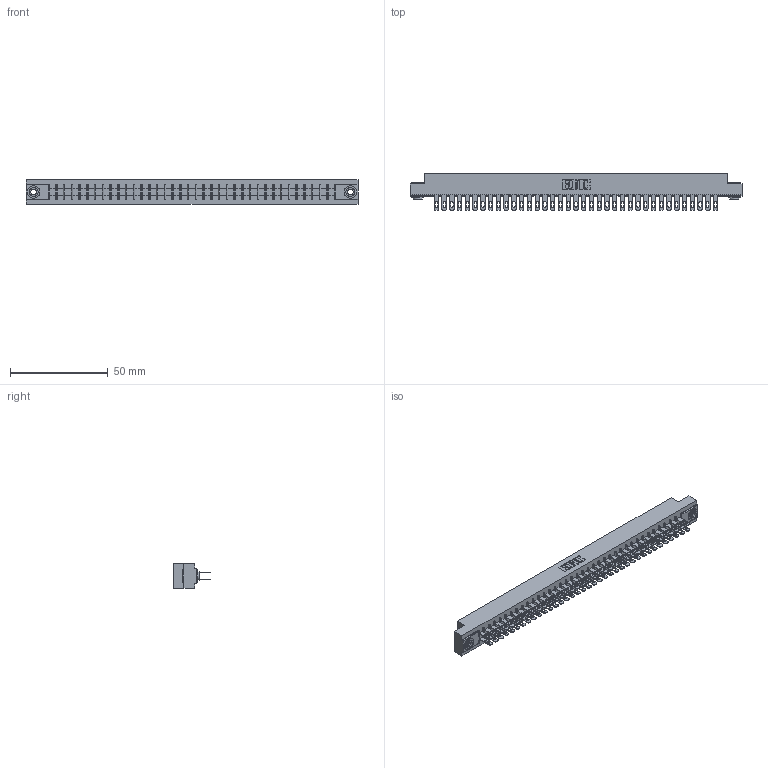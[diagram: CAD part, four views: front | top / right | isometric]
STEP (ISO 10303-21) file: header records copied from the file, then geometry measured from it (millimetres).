
FILE_DESCRIPTION (( 'STEP AP203' ), '1' );
FILE_NAME ('315-074-500-203.STEP', '2019-09-10T21:59:41', ( '' ), ( '' ), 'SwSTEP 2.0', 'SolidWorks 2016', '' );
FILE_SCHEMA (( 'CONFIG_CONTROL_DESIGN' ));
Length unit declared in the file: inch
Products named in the file (4): 305 Part_.156 Dia; 345-250-002_345-250-002-102; 305-290-001_500; 315-074-500-203
Assembly tree (77 placements, depth 2):
  315-074-500-203
    305 Part_.156 Dia
    305-290-001_500  x74
    345-250-002_345-250-002-102  x2
Bounding box: 169.62 x 18.85 x 12.7 mm (x, y, z)
Volume: 17897.6 mm3; surface area: 24349.3 mm2
Topology: 77 solids, 77 shells, 3868 faces, 11047 edges, 7162 vertices
Faces by surface type: plane 2164, cylinder 1548, sphere 148, cone 8
Entity records: 41757 total; most frequent: CARTESIAN_POINT 6890, ORIENTED_EDGE 6830, DIRECTION 6687, EDGE_CURVE 3415, LINE 2745, VECTOR 2745, VERTEX_POINT 2174, AXIS2_PLACEMENT_3D 1971
